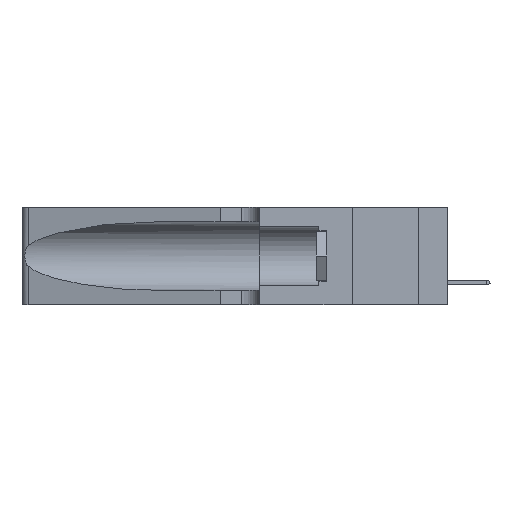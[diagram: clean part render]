
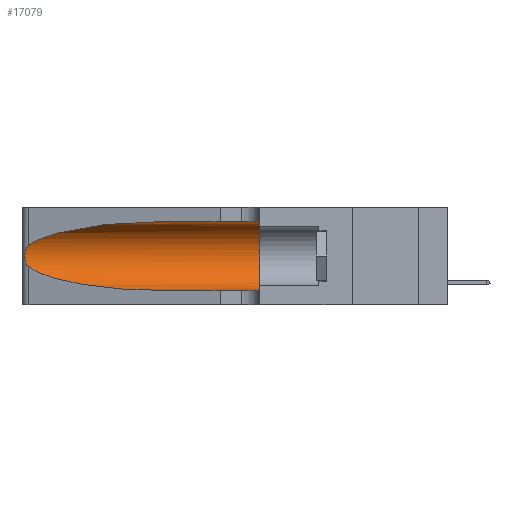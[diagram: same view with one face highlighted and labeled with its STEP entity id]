
A CAD part, left-side view. The second image highlights one B-rep face of the part: STEP entity #17079.
In plain terms, the highlighted cylindrical face has radius 3.308 mm (diameter 6.617 mm), a partial arc.
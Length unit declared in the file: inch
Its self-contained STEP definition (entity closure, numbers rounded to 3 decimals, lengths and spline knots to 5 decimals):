
#1127 = B_SPLINE_CURVE_WITH_KNOTS ( 'NONE', 3,
 ( #18689, #23494, #21019, #14192, #8981, #13980, #4167, #23596, #9089, #28486, #11418, #23699, #28378, #14083 ),
 .UNSPECIFIED., .F., .F.,
 ( 4, 2, 2, 2, 2, 2, 4 ),
 ( 0., 0.00027, 0.00053, 0.00107, 0.0016, 0.00187, 0.00214 ),
 .UNSPECIFIED. ) ;
#1868 = EDGE_CURVE ( 'NONE', #17628, #30184, #11064, .T. ) ;
#1932 = VERTEX_POINT ( 'NONE', #26495 ) ;
#2616 = VERTEX_POINT ( 'NONE', #17850 ) ;
#3263 = LINE ( 'NONE', #17711, #13602 ) ;
#3887 = VERTEX_POINT ( 'NONE', #19194 ) ;
#3908 = CARTESIAN_POINT ( 'NONE',  ( 0.25487, 1.22718, 0.14631 ) ) ;
#4167 = CARTESIAN_POINT ( 'NONE',  ( 0.26075, 1.23896, 0.19203 ) ) ;
#4302 = CARTESIAN_POINT ( 'NONE',  ( 0.18966, 0.96281, 0.05475 ) ) ;
#6895 = CARTESIAN_POINT ( 'NONE',  ( 0.1305, 0.72297, 0.31525 ) ) ;
#7624 = EDGE_CURVE ( 'NONE', #30184, #21648, #3263, .T. ) ;
#7760 = EDGE_CURVE ( 'NONE', #1932, #3887, #27589, .T. ) ;
#8981 = CARTESIAN_POINT ( 'NONE',  ( 0.25854, 1.2359, 0.20912 ) ) ;
#9089 = CARTESIAN_POINT ( 'NONE',  ( 0.26017, 1.23833, 0.17102 ) ) ;
#10124 = DIRECTION ( 'NONE',  ( 0., -1., 0. ) ) ;
#10705 = ORIENTED_EDGE ( 'NONE', *, *, #10797, .T. ) ;
#10797 = EDGE_CURVE ( 'NONE', #3887, #17628, #1127, .T. ) ;
#11064 =( BOUNDED_CURVE ( )  B_SPLINE_CURVE ( 3, ( #21167, #21504, #4302, #26181 ),
 .UNSPECIFIED., .F., .F. ) 
 B_SPLINE_CURVE_WITH_KNOTS ( ( 4, 4 ),
 ( 3.44316, 4.71239 ),
 .UNSPECIFIED. ) 
 CURVE ( )  GEOMETRIC_REPRESENTATION_ITEM ( )  RATIONAL_B_SPLINE_CURVE ( ( 1., 0.87, 0.87, 1. ) ) 
 REPRESENTATION_ITEM ( '' )  );
#11345 = CYLINDRICAL_SURFACE ( 'NONE', #21686, 0.13025 ) ;
#11418 = CARTESIAN_POINT ( 'NONE',  ( 0.25789, 1.23486, 0.15765 ) ) ;
#12287 = DIRECTION ( 'NONE',  ( 0., 0., 1. ) ) ;
#12793 = CARTESIAN_POINT ( 'NONE',  ( 0.1305, 1.61858, 0.185 ) ) ;
#13602 = VECTOR ( 'NONE', #24728, 39.37008 ) ;
#13980 = CARTESIAN_POINT ( 'NONE',  ( 0.26018, 1.23835, 0.19895 ) ) ;
#14083 = CARTESIAN_POINT ( 'NONE',  ( 0.25487, 1.22718, 0.14631 ) ) ;
#14192 = CARTESIAN_POINT ( 'NONE',  ( 0.25787, 1.23484, 0.2124 ) ) ;
#16419 = CARTESIAN_POINT ( 'NONE',  ( 0.18966, 0.96281, 0.31525 ) ) ;
#16498 = DIRECTION ( 'NONE',  ( 0., 1., 0. ) ) ;
#16630 = CARTESIAN_POINT ( 'NONE',  ( 0.25487, 1.22718, 0.22369 ) ) ;
#16643 = EDGE_LOOP ( 'NONE', ( #19587, #10705, #17556, #17775, #20889, #30891 ) ) ;
#17016 = FACE_OUTER_BOUND ( 'NONE', #16643, .T. ) ;
#17079 = ADVANCED_FACE ( 'NONE', ( #17016 ), #11345, .F. ) ;
#17259 = AXIS2_PLACEMENT_3D ( 'NONE', #31075, #16498, #12287 ) ;
#17556 = ORIENTED_EDGE ( 'NONE', *, *, #1868, .T. ) ;
#17624 = DIRECTION ( 'NONE',  ( 0., 0., -1. ) ) ;
#17628 = VERTEX_POINT ( 'NONE', #3908 ) ;
#17711 = CARTESIAN_POINT ( 'NONE',  ( 0.1305, 1.61858, 0.05475 ) ) ;
#17775 = ORIENTED_EDGE ( 'NONE', *, *, #7624, .T. ) ;
#17850 = CARTESIAN_POINT ( 'NONE',  ( 0.1305, 0.35, 0.31525 ) ) ;
#18341 = EDGE_CURVE ( 'NONE', #2616, #21648, #26451, .T. ) ;
#18689 = CARTESIAN_POINT ( 'NONE',  ( 0.25487, 1.22718, 0.22369 ) ) ;
#18775 = DIRECTION ( 'NONE',  ( 0., -1., 0. ) ) ;
#19194 = CARTESIAN_POINT ( 'NONE',  ( 0.25487, 1.22718, 0.22369 ) ) ;
#19377 = VECTOR ( 'NONE', #18775, 39.37008 ) ;
#19587 = ORIENTED_EDGE ( 'NONE', *, *, #7760, .T. ) ;
#20889 = ORIENTED_EDGE ( 'NONE', *, *, #18341, .F. ) ;
#21019 = CARTESIAN_POINT ( 'NONE',  ( 0.25639, 1.23184, 0.21858 ) ) ;
#21167 = CARTESIAN_POINT ( 'NONE',  ( 0.25487, 1.22718, 0.14631 ) ) ;
#21499 = CARTESIAN_POINT ( 'NONE',  ( 0.1305, 0.72297, 0.05475 ) ) ;
#21504 = CARTESIAN_POINT ( 'NONE',  ( 0.2373, 1.15595, 0.08982 ) ) ;
#21648 = VERTEX_POINT ( 'NONE', #23893 ) ;
#21686 = AXIS2_PLACEMENT_3D ( 'NONE', #12793, #10124, #17624 ) ;
#23494 = CARTESIAN_POINT ( 'NONE',  ( 0.25555, 1.22994, 0.2215 ) ) ;
#23596 = CARTESIAN_POINT ( 'NONE',  ( 0.26075, 1.23896, 0.178 ) ) ;
#23699 = CARTESIAN_POINT ( 'NONE',  ( 0.25639, 1.23186, 0.15144 ) ) ;
#23893 = CARTESIAN_POINT ( 'NONE',  ( 0.1305, 0.35, 0.05475 ) ) ;
#24062 = CARTESIAN_POINT ( 'NONE',  ( 0.2373, 1.15595, 0.28018 ) ) ;
#24728 = DIRECTION ( 'NONE',  ( 0., -1., 0. ) ) ;
#26181 = CARTESIAN_POINT ( 'NONE',  ( 0.1305, 0.72297, 0.05475 ) ) ;
#26451 = CIRCLE ( 'NONE', #17259, 0.13025 ) ;
#26495 = CARTESIAN_POINT ( 'NONE',  ( 0.1305, 0.72297, 0.31525 ) ) ;
#27589 =( BOUNDED_CURVE ( )  B_SPLINE_CURVE ( 3, ( #6895, #16419, #24062, #16630 ),
 .UNSPECIFIED., .F., .F. ) 
 B_SPLINE_CURVE_WITH_KNOTS ( ( 4, 4 ),
 ( 1.5708, 2.84003 ),
 .UNSPECIFIED. ) 
 CURVE ( )  GEOMETRIC_REPRESENTATION_ITEM ( )  RATIONAL_B_SPLINE_CURVE ( ( 1., 0.87, 0.87, 1. ) ) 
 REPRESENTATION_ITEM ( '' )  );
#28378 = CARTESIAN_POINT ( 'NONE',  ( 0.25555, 1.22993, 0.14849 ) ) ;
#28486 = CARTESIAN_POINT ( 'NONE',  ( 0.25856, 1.23593, 0.16098 ) ) ;
#28892 = EDGE_CURVE ( 'NONE', #1932, #2616, #29274, .T. ) ;
#29274 = LINE ( 'NONE', #30908, #19377 ) ;
#30184 = VERTEX_POINT ( 'NONE', #21499 ) ;
#30891 = ORIENTED_EDGE ( 'NONE', *, *, #28892, .F. ) ;
#30908 = CARTESIAN_POINT ( 'NONE',  ( 0.1305, 1.61858, 0.31525 ) ) ;
#31075 = CARTESIAN_POINT ( 'NONE',  ( 0.1305, 0.35, 0.185 ) ) ;
